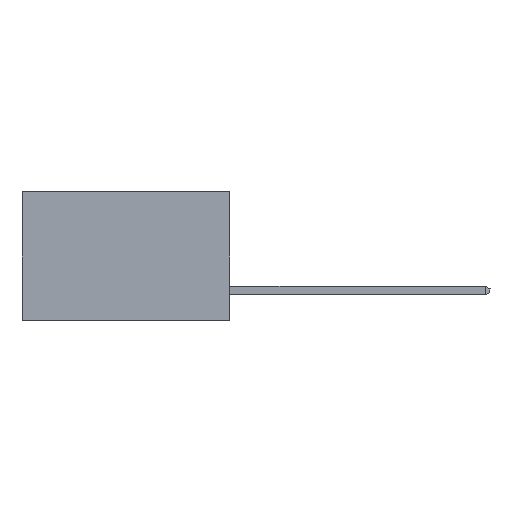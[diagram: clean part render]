
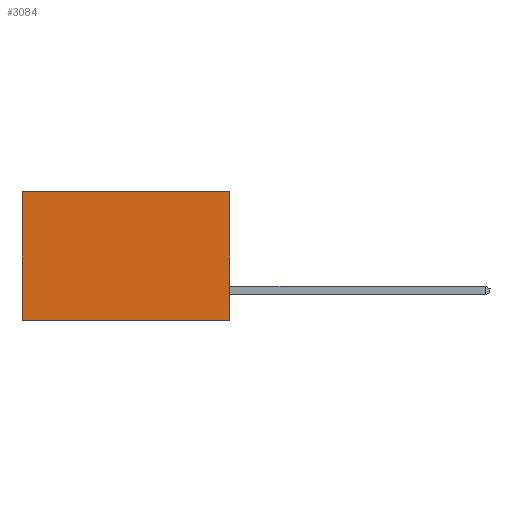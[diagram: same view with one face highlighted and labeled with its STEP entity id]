
A CAD part, left-side view. The second image highlights one B-rep face of the part: STEP entity #3084.
In plain terms, the highlighted planar face has unit normal (-1, 0, 0).
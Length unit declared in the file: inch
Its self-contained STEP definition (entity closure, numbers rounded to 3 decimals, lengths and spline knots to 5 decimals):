
#138 = VERTEX_POINT ( 'NONE', #3169 ) ;
#209 = EDGE_CURVE ( 'NONE', #2270, #9037, #7628, .T. ) ;
#279 = LINE ( 'NONE', #6404, #4668 ) ;
#427 = CARTESIAN_POINT ( 'NONE',  ( 0.2615, 0., 0. ) ) ;
#488 = EDGE_CURVE ( 'NONE', #138, #2270, #279, .T. ) ;
#664 = EDGE_LOOP ( 'NONE', ( #8840, #3549, #6554, #3346 ) ) ;
#774 = PLANE ( 'NONE',  #8566 ) ;
#1702 = DIRECTION ( 'NONE',  ( 0., 0., -1. ) ) ;
#1712 = DIRECTION ( 'NONE',  ( 0., 0., -1. ) ) ;
#2270 = VERTEX_POINT ( 'NONE', #4790 ) ;
#2342 = CARTESIAN_POINT ( 'NONE',  ( 0.2615, 0., -0.37 ) ) ;
#2832 = CARTESIAN_POINT ( 'NONE',  ( 0.2615, 0.6, 0. ) ) ;
#3084 = ADVANCED_FACE ( 'NONE', ( #3199 ), #774, .F. ) ;
#3169 = CARTESIAN_POINT ( 'NONE',  ( 0.2615, 0., 0. ) ) ;
#3199 = FACE_OUTER_BOUND ( 'NONE', #664, .T. ) ;
#3346 = ORIENTED_EDGE ( 'NONE', *, *, #6272, .T. ) ;
#3549 = ORIENTED_EDGE ( 'NONE', *, *, #209, .F. ) ;
#3971 = DIRECTION ( 'NONE',  ( 0., 0., -1. ) ) ;
#3979 = VECTOR ( 'NONE', #3971, 39.37008 ) ;
#4668 = VECTOR ( 'NONE', #1702, 39.37008 ) ;
#4790 = CARTESIAN_POINT ( 'NONE',  ( 0.2615, 0., -0.37 ) ) ;
#6271 = LINE ( 'NONE', #8629, #3979 ) ;
#6272 = EDGE_CURVE ( 'NONE', #138, #6713, #8380, .T. ) ;
#6345 = VECTOR ( 'NONE', #10004, 39.37008 ) ;
#6404 = CARTESIAN_POINT ( 'NONE',  ( 0.2615, 0., -0.37 ) ) ;
#6554 = ORIENTED_EDGE ( 'NONE', *, *, #488, .F. ) ;
#6713 = VERTEX_POINT ( 'NONE', #2832 ) ;
#7274 = CARTESIAN_POINT ( 'NONE',  ( 0.2615, 0.6, -0.37 ) ) ;
#7628 = LINE ( 'NONE', #9286, #6345 ) ;
#8380 = LINE ( 'NONE', #427, #10064 ) ;
#8459 = EDGE_CURVE ( 'NONE', #6713, #9037, #6271, .T. ) ;
#8566 = AXIS2_PLACEMENT_3D ( 'NONE', #2342, #9577, #1712 ) ;
#8629 = CARTESIAN_POINT ( 'NONE',  ( 0.2615, 0.6, -0.37 ) ) ;
#8840 = ORIENTED_EDGE ( 'NONE', *, *, #8459, .T. ) ;
#9037 = VERTEX_POINT ( 'NONE', #7274 ) ;
#9286 = CARTESIAN_POINT ( 'NONE',  ( 0.2615, 0., -0.37 ) ) ;
#9310 = DIRECTION ( 'NONE',  ( 0., 1., 0. ) ) ;
#9577 = DIRECTION ( 'NONE',  ( 1., 0., 0. ) ) ;
#10004 = DIRECTION ( 'NONE',  ( 0., 1., 0. ) ) ;
#10064 = VECTOR ( 'NONE', #9310, 39.37008 ) ;
